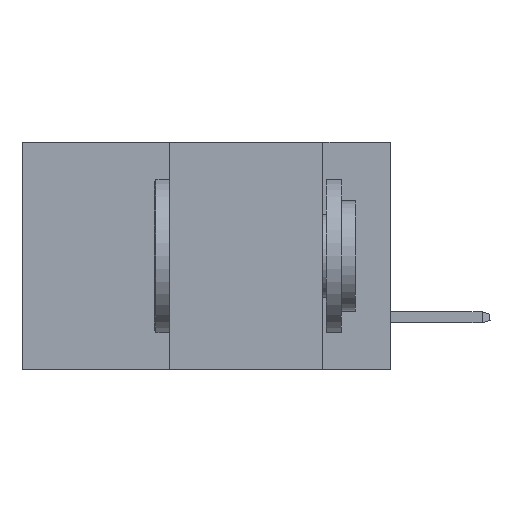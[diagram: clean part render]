
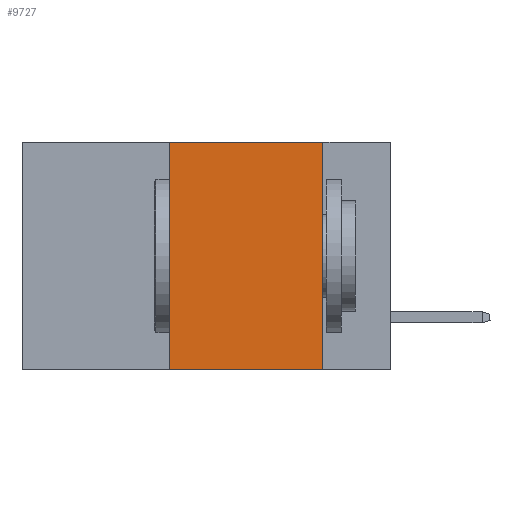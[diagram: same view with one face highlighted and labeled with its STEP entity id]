
A CAD part, left-side view. The second image highlights one B-rep face of the part: STEP entity #9727.
In plain terms, the highlighted planar face has unit normal (-1, 0, 0).
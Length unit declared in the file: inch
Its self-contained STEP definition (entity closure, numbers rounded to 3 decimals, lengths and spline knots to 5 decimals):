
#894 = CARTESIAN_POINT ( 'NONE',  ( 0., 0.36, -0.37 ) ) ;
#2870 = EDGE_LOOP ( 'NONE', ( #35793, #10275, #35454, #7249 ) ) ;
#7249 = ORIENTED_EDGE ( 'NONE', *, *, #20612, .T. ) ;
#7824 = DIRECTION ( 'NONE',  ( 1., 0., 0. ) ) ;
#8605 = LINE ( 'NONE', #16073, #14466 ) ;
#9727 = ADVANCED_FACE ( 'NONE', ( #17650 ), #30730, .F. ) ;
#10275 = ORIENTED_EDGE ( 'NONE', *, *, #46404, .F. ) ;
#11412 = DIRECTION ( 'NONE',  ( 0., -1., 0. ) ) ;
#11778 = DIRECTION ( 'NONE',  ( 0., 0., -1. ) ) ;
#12100 = DIRECTION ( 'NONE',  ( 0., -1., 0. ) ) ;
#14466 = VECTOR ( 'NONE', #12100, 39.37008 ) ;
#16073 = CARTESIAN_POINT ( 'NONE',  ( 0., 0.6, -0.37 ) ) ;
#17650 = FACE_OUTER_BOUND ( 'NONE', #2870, .T. ) ;
#20612 = EDGE_CURVE ( 'NONE', #44023, #33502, #8605, .T. ) ;
#20895 = CARTESIAN_POINT ( 'NONE',  ( 0., 0.36, 0. ) ) ;
#21902 = DIRECTION ( 'NONE',  ( 0., 0., 1. ) ) ;
#22689 = DIRECTION ( 'NONE',  ( 0., 0., -1. ) ) ;
#24370 = VECTOR ( 'NONE', #11412, 39.37008 ) ;
#30730 = PLANE ( 'NONE',  #38394 ) ;
#31092 = VECTOR ( 'NONE', #22689, 39.37008 ) ;
#31909 = EDGE_CURVE ( 'NONE', #35903, #33502, #37033, .T. ) ;
#32080 = LINE ( 'NONE', #45648, #24370 ) ;
#32854 = CARTESIAN_POINT ( 'NONE',  ( 0., 0.11, 0. ) ) ;
#33502 = VERTEX_POINT ( 'NONE', #38832 ) ;
#35454 = ORIENTED_EDGE ( 'NONE', *, *, #46313, .F. ) ;
#35793 = ORIENTED_EDGE ( 'NONE', *, *, #31909, .F. ) ;
#35903 = VERTEX_POINT ( 'NONE', #32854 ) ;
#36264 = VECTOR ( 'NONE', #21902, 39.37008 ) ;
#36889 = VERTEX_POINT ( 'NONE', #20895 ) ;
#37033 = LINE ( 'NONE', #44946, #31092 ) ;
#38394 = AXIS2_PLACEMENT_3D ( 'NONE', #48989, #7824, #11778 ) ;
#38832 = CARTESIAN_POINT ( 'NONE',  ( 0., 0.11, -0.37 ) ) ;
#44023 = VERTEX_POINT ( 'NONE', #894 ) ;
#44946 = CARTESIAN_POINT ( 'NONE',  ( 0., 0.11, 0. ) ) ;
#45648 = CARTESIAN_POINT ( 'NONE',  ( 0., 0.6, 0. ) ) ;
#46313 = EDGE_CURVE ( 'NONE', #44023, #36889, #46388, .T. ) ;
#46388 = LINE ( 'NONE', #47957, #36264 ) ;
#46404 = EDGE_CURVE ( 'NONE', #36889, #35903, #32080, .T. ) ;
#47957 = CARTESIAN_POINT ( 'NONE',  ( 0., 0.36, 0. ) ) ;
#48989 = CARTESIAN_POINT ( 'NONE',  ( 0., 0.6, 0. ) ) ;
